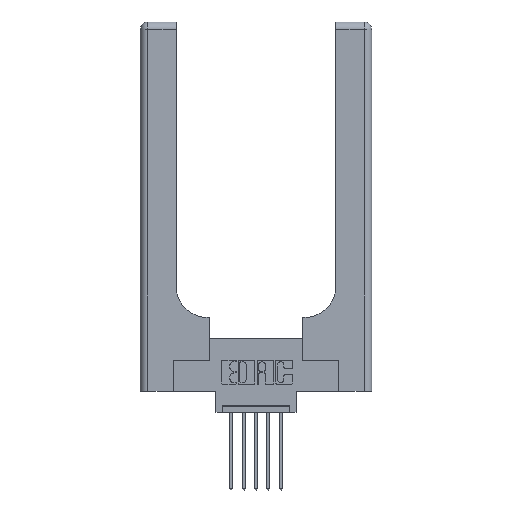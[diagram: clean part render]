
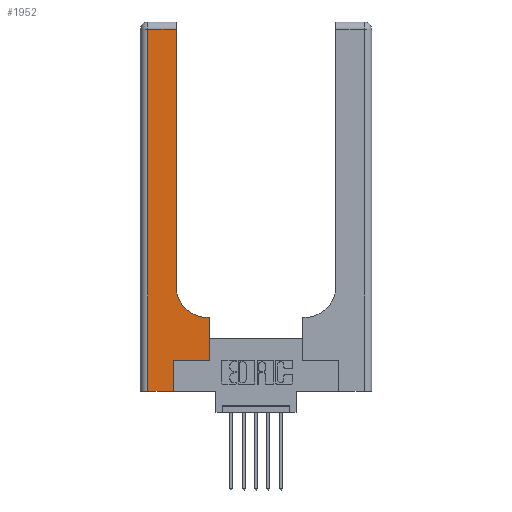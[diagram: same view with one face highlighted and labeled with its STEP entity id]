
A CAD part, top view. The second image highlights one B-rep face of the part: STEP entity #1952.
In plain terms, the highlighted planar face has unit normal (0, 0, 1).
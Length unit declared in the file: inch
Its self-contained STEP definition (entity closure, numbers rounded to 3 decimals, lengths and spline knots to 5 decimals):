
#176 = CARTESIAN_POINT ( 'NONE',  ( 0.2915, 0.85, 0.37 ) ) ;
#688 = AXIS2_PLACEMENT_3D ( 'NONE', #10994, #2176, #3377 ) ;
#827 = DIRECTION ( 'NONE',  ( 0., 1., 0. ) ) ;
#974 = DIRECTION ( 'NONE',  ( 0., 1., 0. ) ) ;
#1021 = LINE ( 'NONE', #4194, #2030 ) ;
#1189 = LINE ( 'NONE', #3454, #12467 ) ;
#1488 = CARTESIAN_POINT ( 'NONE',  ( 0.269, 0.25, 0.37 ) ) ;
#1652 = FACE_OUTER_BOUND ( 'NONE', #1772, .T. ) ;
#1772 = EDGE_LOOP ( 'NONE', ( #11857, #13235, #6434, #8878, #3267, #4798, #9376, #4118, #5644 ) ) ;
#1796 = VECTOR ( 'NONE', #5939, 39.37008 ) ;
#1836 = CARTESIAN_POINT ( 'NONE',  ( 0., 0., 0.37 ) ) ;
#1952 = ADVANCED_FACE ( 'NONE', ( #1652 ), #8845, .F. ) ;
#2030 = VECTOR ( 'NONE', #974, 39.37008 ) ;
#2116 = AXIS2_PLACEMENT_3D ( 'NONE', #5679, #5620, #12160 ) ;
#2176 = DIRECTION ( 'NONE',  ( 0., 0., -1. ) ) ;
#2207 = CARTESIAN_POINT ( 'NONE',  ( 0.2915, 2.94, 0.37 ) ) ;
#2287 = VERTEX_POINT ( 'NONE', #10166 ) ;
#2443 = VERTEX_POINT ( 'NONE', #176 ) ;
#2477 = CARTESIAN_POINT ( 'NONE',  ( 0.5585, 0.25, 0.37 ) ) ;
#2543 = DIRECTION ( 'NONE',  ( -1., 0., 0. ) ) ;
#2824 = EDGE_CURVE ( 'NONE', #6838, #12671, #11866, .T. ) ;
#2850 = VECTOR ( 'NONE', #827, 39.37008 ) ;
#3121 = CARTESIAN_POINT ( 'NONE',  ( 0.5585, 0.6, 0.37 ) ) ;
#3267 = ORIENTED_EDGE ( 'NONE', *, *, #10241, .T. ) ;
#3377 = DIRECTION ( 'NONE',  ( -1., 0., 0. ) ) ;
#3454 = CARTESIAN_POINT ( 'NONE',  ( 0., 2.94, 0.37 ) ) ;
#3893 = CARTESIAN_POINT ( 'NONE',  ( 0.269, 0.25, 0.37 ) ) ;
#4118 = ORIENTED_EDGE ( 'NONE', *, *, #2824, .T. ) ;
#4194 = CARTESIAN_POINT ( 'NONE',  ( 0.5585, 0.25, 0.37 ) ) ;
#4230 = DIRECTION ( 'NONE',  ( 0., -1., 0. ) ) ;
#4469 = CARTESIAN_POINT ( 'NONE',  ( 0.06, 2.94, 0.37 ) ) ;
#4798 = ORIENTED_EDGE ( 'NONE', *, *, #7797, .T. ) ;
#5018 = CARTESIAN_POINT ( 'NONE',  ( 0.269, 0., 0.37 ) ) ;
#5620 = DIRECTION ( 'NONE',  ( 0., 0., -1. ) ) ;
#5644 = ORIENTED_EDGE ( 'NONE', *, *, #8683, .T. ) ;
#5679 = CARTESIAN_POINT ( 'NONE',  ( 0.5415, 0.85, 0.37 ) ) ;
#5892 = CARTESIAN_POINT ( 'NONE',  ( 0.5415, 0.6, 0.37 ) ) ;
#5939 = DIRECTION ( 'NONE',  ( 1., 0., 0. ) ) ;
#6147 = EDGE_CURVE ( 'NONE', #8229, #6838, #1021, .T. ) ;
#6157 = DIRECTION ( 'NONE',  ( 0., 1., 0. ) ) ;
#6434 = ORIENTED_EDGE ( 'NONE', *, *, #8589, .T. ) ;
#6752 = LINE ( 'NONE', #7604, #7102 ) ;
#6838 = VERTEX_POINT ( 'NONE', #3121 ) ;
#6917 = EDGE_CURVE ( 'NONE', #2443, #12270, #8150, .T. ) ;
#6969 = CARTESIAN_POINT ( 'NONE',  ( 0.06, 0., 0.37 ) ) ;
#7102 = VECTOR ( 'NONE', #4230, 39.37008 ) ;
#7604 = CARTESIAN_POINT ( 'NONE',  ( 0.06, 3., 0.37 ) ) ;
#7650 = VECTOR ( 'NONE', #12904, 39.37008 ) ;
#7797 = EDGE_CURVE ( 'NONE', #13109, #8229, #10142, .T. ) ;
#8150 = LINE ( 'NONE', #13013, #2850 ) ;
#8164 = VERTEX_POINT ( 'NONE', #6969 ) ;
#8180 = LINE ( 'NONE', #1836, #7650 ) ;
#8229 = VERTEX_POINT ( 'NONE', #2477 ) ;
#8589 = EDGE_CURVE ( 'NONE', #10501, #8164, #6752, .T. ) ;
#8683 = EDGE_CURVE ( 'NONE', #12671, #2443, #13405, .T. ) ;
#8731 = LINE ( 'NONE', #5018, #11135 ) ;
#8845 = PLANE ( 'NONE',  #688 ) ;
#8878 = ORIENTED_EDGE ( 'NONE', *, *, #12193, .T. ) ;
#9376 = ORIENTED_EDGE ( 'NONE', *, *, #6147, .T. ) ;
#10030 = CARTESIAN_POINT ( 'NONE',  ( 0.2915, 0.6, 0.37 ) ) ;
#10142 = LINE ( 'NONE', #3893, #1796 ) ;
#10166 = CARTESIAN_POINT ( 'NONE',  ( 0.269, 0., 0.37 ) ) ;
#10241 = EDGE_CURVE ( 'NONE', #2287, #13109, #8731, .T. ) ;
#10501 = VERTEX_POINT ( 'NONE', #4469 ) ;
#10994 = CARTESIAN_POINT ( 'NONE',  ( 0., 3., 0.37 ) ) ;
#11135 = VECTOR ( 'NONE', #6157, 39.37008 ) ;
#11536 = VECTOR ( 'NONE', #2543, 39.37008 ) ;
#11857 = ORIENTED_EDGE ( 'NONE', *, *, #6917, .T. ) ;
#11866 = LINE ( 'NONE', #10030, #11536 ) ;
#12160 = DIRECTION ( 'NONE',  ( 1., 0., 0. ) ) ;
#12193 = EDGE_CURVE ( 'NONE', #8164, #2287, #8180, .T. ) ;
#12270 = VERTEX_POINT ( 'NONE', #2207 ) ;
#12467 = VECTOR ( 'NONE', #13188, 39.37008 ) ;
#12512 = EDGE_CURVE ( 'NONE', #12270, #10501, #1189, .T. ) ;
#12671 = VERTEX_POINT ( 'NONE', #5892 ) ;
#12904 = DIRECTION ( 'NONE',  ( 1., 0., 0. ) ) ;
#13013 = CARTESIAN_POINT ( 'NONE',  ( 0.2915, 3., 0.37 ) ) ;
#13109 = VERTEX_POINT ( 'NONE', #1488 ) ;
#13188 = DIRECTION ( 'NONE',  ( -1., 0., 0. ) ) ;
#13235 = ORIENTED_EDGE ( 'NONE', *, *, #12512, .T. ) ;
#13405 = CIRCLE ( 'NONE', #2116, 0.25 ) ;
